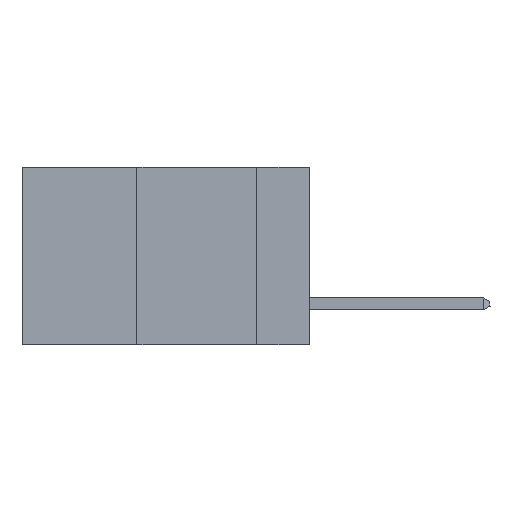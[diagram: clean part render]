
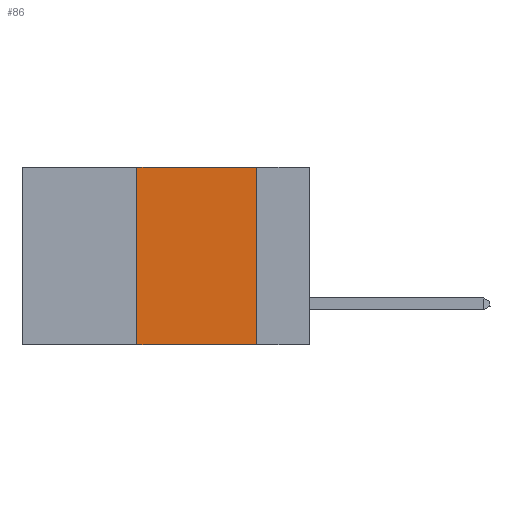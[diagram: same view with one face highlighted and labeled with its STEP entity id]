
A CAD part, left-side view. The second image highlights one B-rep face of the part: STEP entity #86.
In plain terms, the highlighted planar face has unit normal (-1, 0, 0).
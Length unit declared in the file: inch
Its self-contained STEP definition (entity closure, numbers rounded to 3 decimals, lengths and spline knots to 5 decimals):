
#86 = ADVANCED_FACE ( 'NONE', ( #4940 ), #18326, .F. ) ;
#172 = VECTOR ( 'NONE', #37254, 39.37008 ) ;
#550 = CARTESIAN_POINT ( 'NONE',  ( 0., 0.11, 0. ) ) ;
#2585 = EDGE_CURVE ( 'NONE', #9110, #26810, #11142, .T. ) ;
#2645 = CARTESIAN_POINT ( 'NONE',  ( 0., 0.6, 0. ) ) ;
#3033 = CARTESIAN_POINT ( 'NONE',  ( 0., 0.36, 0. ) ) ;
#4940 = FACE_OUTER_BOUND ( 'NONE', #30154, .T. ) ;
#5662 = ORIENTED_EDGE ( 'NONE', *, *, #32129, .F. ) ;
#6439 = LINE ( 'NONE', #2645, #40499 ) ;
#7664 = CARTESIAN_POINT ( 'NONE',  ( 0., 0.11, -0.37 ) ) ;
#9110 = VERTEX_POINT ( 'NONE', #10154 ) ;
#10154 = CARTESIAN_POINT ( 'NONE',  ( 0., 0.36, -0.37 ) ) ;
#11142 = LINE ( 'NONE', #43265, #25727 ) ;
#13119 = CARTESIAN_POINT ( 'NONE',  ( 0., 0.11, 0. ) ) ;
#15130 = EDGE_CURVE ( 'NONE', #31614, #40502, #6439, .T. ) ;
#18326 = PLANE ( 'NONE',  #41432 ) ;
#18590 = LINE ( 'NONE', #13119, #172 ) ;
#20412 = VECTOR ( 'NONE', #27345, 39.37008 ) ;
#22974 = ORIENTED_EDGE ( 'NONE', *, *, #25940, .F. ) ;
#24055 = DIRECTION ( 'NONE',  ( 0., -1., 0. ) ) ;
#25727 = VECTOR ( 'NONE', #24055, 39.37008 ) ;
#25940 = EDGE_CURVE ( 'NONE', #9110, #31614, #27347, .T. ) ;
#26808 = DIRECTION ( 'NONE',  ( 0., -1., 0. ) ) ;
#26810 = VERTEX_POINT ( 'NONE', #7664 ) ;
#27345 = DIRECTION ( 'NONE',  ( 0., 0., 1. ) ) ;
#27347 = LINE ( 'NONE', #33998, #20412 ) ;
#30154 = EDGE_LOOP ( 'NONE', ( #5662, #31704, #22974, #33782 ) ) ;
#31614 = VERTEX_POINT ( 'NONE', #3033 ) ;
#31704 = ORIENTED_EDGE ( 'NONE', *, *, #15130, .F. ) ;
#32129 = EDGE_CURVE ( 'NONE', #40502, #26810, #18590, .T. ) ;
#32649 = DIRECTION ( 'NONE',  ( 0., 0., -1. ) ) ;
#33782 = ORIENTED_EDGE ( 'NONE', *, *, #2585, .T. ) ;
#33998 = CARTESIAN_POINT ( 'NONE',  ( 0., 0.36, 0. ) ) ;
#35664 = CARTESIAN_POINT ( 'NONE',  ( 0., 0.6, 0. ) ) ;
#37254 = DIRECTION ( 'NONE',  ( 0., 0., -1. ) ) ;
#40499 = VECTOR ( 'NONE', #26808, 39.37008 ) ;
#40502 = VERTEX_POINT ( 'NONE', #550 ) ;
#41432 = AXIS2_PLACEMENT_3D ( 'NONE', #35664, #42611, #32649 ) ;
#42611 = DIRECTION ( 'NONE',  ( 1., 0., 0. ) ) ;
#43265 = CARTESIAN_POINT ( 'NONE',  ( 0., 0.6, -0.37 ) ) ;
